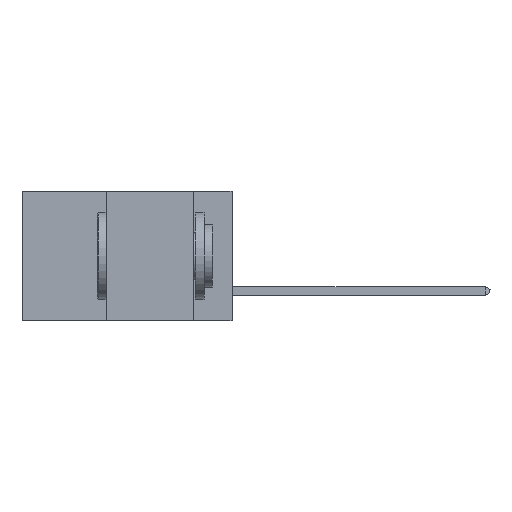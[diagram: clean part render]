
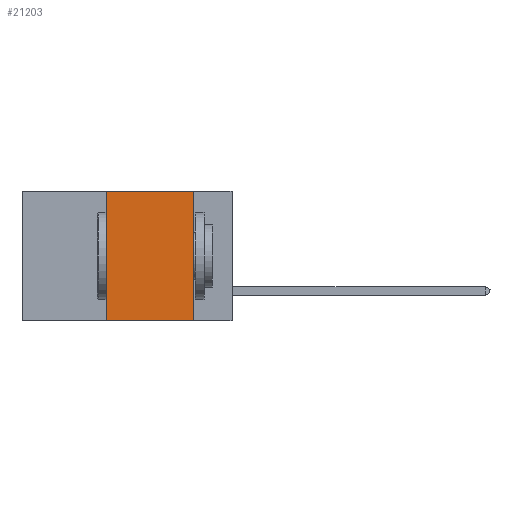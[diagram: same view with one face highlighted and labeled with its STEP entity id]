
A CAD part, left-side view. The second image highlights one B-rep face of the part: STEP entity #21203.
In plain terms, the highlighted planar face has unit normal (-1, 0, 0).
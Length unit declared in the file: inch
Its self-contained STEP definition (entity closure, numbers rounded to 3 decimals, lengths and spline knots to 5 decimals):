
#1443 = ORIENTED_EDGE ( 'NONE', *, *, #35185, .F. ) ;
#2071 = CARTESIAN_POINT ( 'NONE',  ( 0., 0.11, -0.37 ) ) ;
#3105 = DIRECTION ( 'NONE',  ( 0., 0., -1. ) ) ;
#3617 = LINE ( 'NONE', #19374, #41592 ) ;
#4309 = DIRECTION ( 'NONE',  ( 0., 0., 1. ) ) ;
#4503 = ORIENTED_EDGE ( 'NONE', *, *, #32276, .F. ) ;
#7267 = PLANE ( 'NONE',  #12625 ) ;
#7811 = CARTESIAN_POINT ( 'NONE',  ( 0., 0.36, -0.37 ) ) ;
#12525 = VERTEX_POINT ( 'NONE', #2071 ) ;
#12625 = AXIS2_PLACEMENT_3D ( 'NONE', #43489, #17801, #3105 ) ;
#13540 = EDGE_CURVE ( 'NONE', #24321, #12525, #23387, .T. ) ;
#14587 = CARTESIAN_POINT ( 'NONE',  ( 0., 0.6, 0. ) ) ;
#16497 = LINE ( 'NONE', #33518, #47610 ) ;
#17801 = DIRECTION ( 'NONE',  ( 1., 0., 0. ) ) ;
#18777 = VECTOR ( 'NONE', #19762, 39.37008 ) ;
#19374 = CARTESIAN_POINT ( 'NONE',  ( 0., 0.6, -0.37 ) ) ;
#19762 = DIRECTION ( 'NONE',  ( 0., 0., -1. ) ) ;
#21203 = ADVANCED_FACE ( 'NONE', ( #38406 ), #7267, .F. ) ;
#21692 = VERTEX_POINT ( 'NONE', #7811 ) ;
#23387 = LINE ( 'NONE', #44789, #18777 ) ;
#24321 = VERTEX_POINT ( 'NONE', #45457 ) ;
#28815 = EDGE_CURVE ( 'NONE', #21692, #12525, #3617, .T. ) ;
#29786 = DIRECTION ( 'NONE',  ( 0., -1., 0. ) ) ;
#32076 = LINE ( 'NONE', #14587, #45217 ) ;
#32276 = EDGE_CURVE ( 'NONE', #21692, #38010, #16497, .T. ) ;
#33518 = CARTESIAN_POINT ( 'NONE',  ( 0., 0.36, 0. ) ) ;
#35185 = EDGE_CURVE ( 'NONE', #38010, #24321, #32076, .T. ) ;
#36271 = ORIENTED_EDGE ( 'NONE', *, *, #13540, .F. ) ;
#37547 = DIRECTION ( 'NONE',  ( 0., -1., 0. ) ) ;
#38010 = VERTEX_POINT ( 'NONE', #40788 ) ;
#38406 = FACE_OUTER_BOUND ( 'NONE', #45266, .T. ) ;
#39610 = ORIENTED_EDGE ( 'NONE', *, *, #28815, .T. ) ;
#40788 = CARTESIAN_POINT ( 'NONE',  ( 0., 0.36, 0. ) ) ;
#41592 = VECTOR ( 'NONE', #29786, 39.37008 ) ;
#43489 = CARTESIAN_POINT ( 'NONE',  ( 0., 0.6, 0. ) ) ;
#44789 = CARTESIAN_POINT ( 'NONE',  ( 0., 0.11, 0. ) ) ;
#45217 = VECTOR ( 'NONE', #37547, 39.37008 ) ;
#45266 = EDGE_LOOP ( 'NONE', ( #36271, #1443, #4503, #39610 ) ) ;
#45457 = CARTESIAN_POINT ( 'NONE',  ( 0., 0.11, 0. ) ) ;
#47610 = VECTOR ( 'NONE', #4309, 39.37008 ) ;
